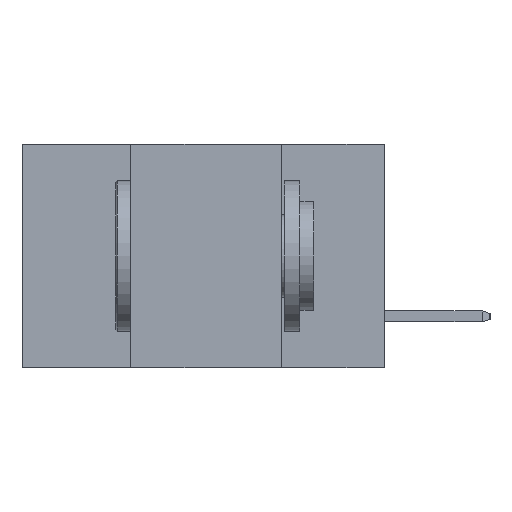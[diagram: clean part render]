
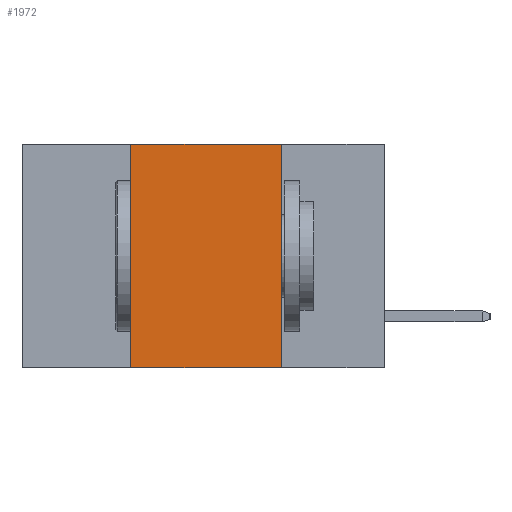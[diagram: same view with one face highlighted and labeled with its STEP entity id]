
A CAD part, left-side view. The second image highlights one B-rep face of the part: STEP entity #1972.
In plain terms, the highlighted planar face has unit normal (-1, 0, 0).
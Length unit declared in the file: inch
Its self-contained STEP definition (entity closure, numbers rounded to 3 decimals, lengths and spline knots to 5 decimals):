
#606 = CARTESIAN_POINT ( 'NONE',  ( 0., 0.17, 0. ) ) ;
#1114 = DIRECTION ( 'NONE',  ( 0., 0., -1. ) ) ;
#1137 = DIRECTION ( 'NONE',  ( 1., 0., 0. ) ) ;
#1187 = CARTESIAN_POINT ( 'NONE',  ( 0., 0.17, -0.37 ) ) ;
#1248 = PLANE ( 'NONE',  #6252 ) ;
#1591 = DIRECTION ( 'NONE',  ( 0., 0., -1. ) ) ;
#1837 = CARTESIAN_POINT ( 'NONE',  ( 0., 0.6, 0. ) ) ;
#1972 = ADVANCED_FACE ( 'NONE', ( #8123 ), #1248, .F. ) ;
#3077 = EDGE_CURVE ( 'NONE', #16664, #3211, #9342, .T. ) ;
#3211 = VERTEX_POINT ( 'NONE', #10965 ) ;
#6237 = VECTOR ( 'NONE', #21380, 39.37008 ) ;
#6252 = AXIS2_PLACEMENT_3D ( 'NONE', #1837, #1137, #1114 ) ;
#6359 = EDGE_LOOP ( 'NONE', ( #9530, #18845, #10811, #9374 ) ) ;
#6732 = VECTOR ( 'NONE', #16783, 39.37008 ) ;
#7080 = EDGE_CURVE ( 'NONE', #16664, #7442, #11200, .T. ) ;
#7442 = VERTEX_POINT ( 'NONE', #14884 ) ;
#8123 = FACE_OUTER_BOUND ( 'NONE', #6359, .T. ) ;
#9342 = LINE ( 'NONE', #15702, #22698 ) ;
#9374 = ORIENTED_EDGE ( 'NONE', *, *, #3077, .T. ) ;
#9530 = ORIENTED_EDGE ( 'NONE', *, *, #16517, .F. ) ;
#10811 = ORIENTED_EDGE ( 'NONE', *, *, #7080, .F. ) ;
#10965 = CARTESIAN_POINT ( 'NONE',  ( 0., 0.17, -0.37 ) ) ;
#11200 = LINE ( 'NONE', #21631, #6237 ) ;
#11732 = LINE ( 'NONE', #17090, #6732 ) ;
#14884 = CARTESIAN_POINT ( 'NONE',  ( 0., 0.42, 0. ) ) ;
#14978 = DIRECTION ( 'NONE',  ( 0., -1., 0. ) ) ;
#15702 = CARTESIAN_POINT ( 'NONE',  ( 0., 0.6, -0.37 ) ) ;
#15894 = EDGE_CURVE ( 'NONE', #7442, #22379, #11732, .T. ) ;
#16517 = EDGE_CURVE ( 'NONE', #22379, #3211, #16926, .T. ) ;
#16664 = VERTEX_POINT ( 'NONE', #20730 ) ;
#16783 = DIRECTION ( 'NONE',  ( 0., -1., 0. ) ) ;
#16926 = LINE ( 'NONE', #1187, #18051 ) ;
#17090 = CARTESIAN_POINT ( 'NONE',  ( 0., 0.6, 0. ) ) ;
#18051 = VECTOR ( 'NONE', #1591, 39.37008 ) ;
#18845 = ORIENTED_EDGE ( 'NONE', *, *, #15894, .F. ) ;
#20730 = CARTESIAN_POINT ( 'NONE',  ( 0., 0.42, -0.37 ) ) ;
#21380 = DIRECTION ( 'NONE',  ( 0., 0., 1. ) ) ;
#21631 = CARTESIAN_POINT ( 'NONE',  ( 0., 0.42, -0.37 ) ) ;
#22379 = VERTEX_POINT ( 'NONE', #606 ) ;
#22698 = VECTOR ( 'NONE', #14978, 39.37008 ) ;
